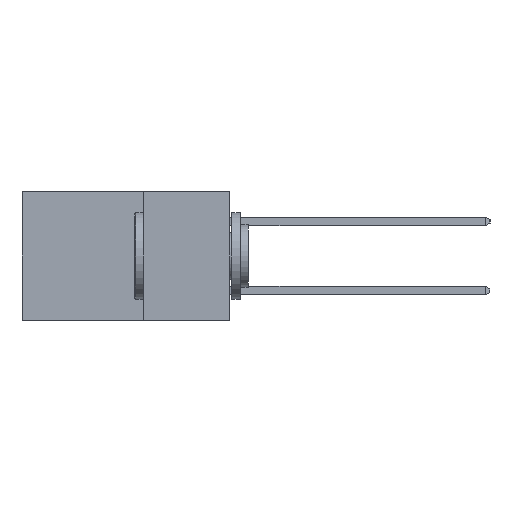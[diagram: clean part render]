
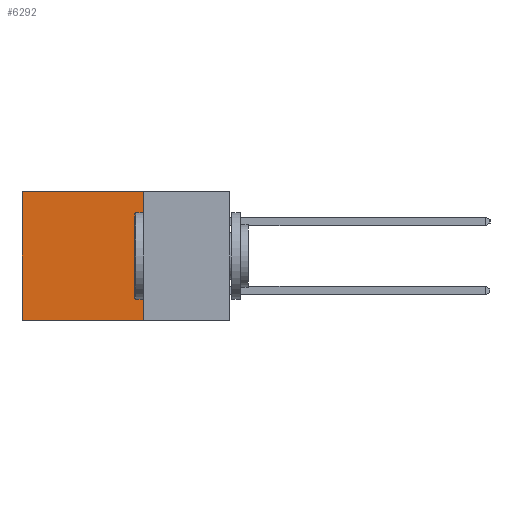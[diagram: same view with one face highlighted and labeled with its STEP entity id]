
A CAD part, left-side view. The second image highlights one B-rep face of the part: STEP entity #6292.
In plain terms, the highlighted planar face has unit normal (-1, 0, 0).
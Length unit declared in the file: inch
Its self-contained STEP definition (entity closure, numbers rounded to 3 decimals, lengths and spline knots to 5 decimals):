
#200 = CARTESIAN_POINT ( 'NONE',  ( 0.298, 0.25, -0.37 ) ) ;
#600 = CARTESIAN_POINT ( 'NONE',  ( 0.298, 0.25, 0. ) ) ;
#761 = VERTEX_POINT ( 'NONE', #1379 ) ;
#1379 = CARTESIAN_POINT ( 'NONE',  ( 0.298, 0.25, -0.37 ) ) ;
#1483 = VECTOR ( 'NONE', #12370, 39.37008 ) ;
#1579 = DIRECTION ( 'NONE',  ( 1., 0., 0. ) ) ;
#1690 = VECTOR ( 'NONE', #5536, 39.37008 ) ;
#1893 = CARTESIAN_POINT ( 'NONE',  ( 0.298, 0.6, 0. ) ) ;
#2886 = EDGE_CURVE ( 'NONE', #11017, #13200, #12539, .T. ) ;
#3175 = VECTOR ( 'NONE', #14532, 39.37008 ) ;
#3835 = EDGE_CURVE ( 'NONE', #13200, #15323, #11935, .T. ) ;
#3946 = AXIS2_PLACEMENT_3D ( 'NONE', #6752, #1579, #10733 ) ;
#4420 = ORIENTED_EDGE ( 'NONE', *, *, #2886, .T. ) ;
#4430 = ORIENTED_EDGE ( 'NONE', *, *, #5084, .F. ) ;
#4528 = FACE_OUTER_BOUND ( 'NONE', #6941, .T. ) ;
#5084 = EDGE_CURVE ( 'NONE', #11017, #761, #5994, .T. ) ;
#5536 = DIRECTION ( 'NONE',  ( 0., 1., 0. ) ) ;
#5994 = LINE ( 'NONE', #7223, #12573 ) ;
#6292 = ADVANCED_FACE ( 'NONE', ( #4528 ), #9417, .F. ) ;
#6656 = LINE ( 'NONE', #200, #3175 ) ;
#6752 = CARTESIAN_POINT ( 'NONE',  ( 0.298, 0.25, 0. ) ) ;
#6941 = EDGE_LOOP ( 'NONE', ( #14542, #9843, #4430, #4420 ) ) ;
#7223 = CARTESIAN_POINT ( 'NONE',  ( 0.298, 0.25, 0. ) ) ;
#8569 = DIRECTION ( 'NONE',  ( 0., 0., -1. ) ) ;
#9417 = PLANE ( 'NONE',  #3946 ) ;
#9843 = ORIENTED_EDGE ( 'NONE', *, *, #16511, .F. ) ;
#10733 = DIRECTION ( 'NONE',  ( 0., 0., -1. ) ) ;
#11017 = VERTEX_POINT ( 'NONE', #600 ) ;
#11935 = LINE ( 'NONE', #1893, #1483 ) ;
#12370 = DIRECTION ( 'NONE',  ( 0., 0., -1. ) ) ;
#12539 = LINE ( 'NONE', #13387, #1690 ) ;
#12573 = VECTOR ( 'NONE', #8569, 39.37008 ) ;
#13200 = VERTEX_POINT ( 'NONE', #13671 ) ;
#13387 = CARTESIAN_POINT ( 'NONE',  ( 0.298, 0.25, 0. ) ) ;
#13671 = CARTESIAN_POINT ( 'NONE',  ( 0.298, 0.6, 0. ) ) ;
#14532 = DIRECTION ( 'NONE',  ( 0., 1., 0. ) ) ;
#14542 = ORIENTED_EDGE ( 'NONE', *, *, #3835, .T. ) ;
#14875 = CARTESIAN_POINT ( 'NONE',  ( 0.298, 0.6, -0.37 ) ) ;
#15323 = VERTEX_POINT ( 'NONE', #14875 ) ;
#16511 = EDGE_CURVE ( 'NONE', #761, #15323, #6656, .T. ) ;
